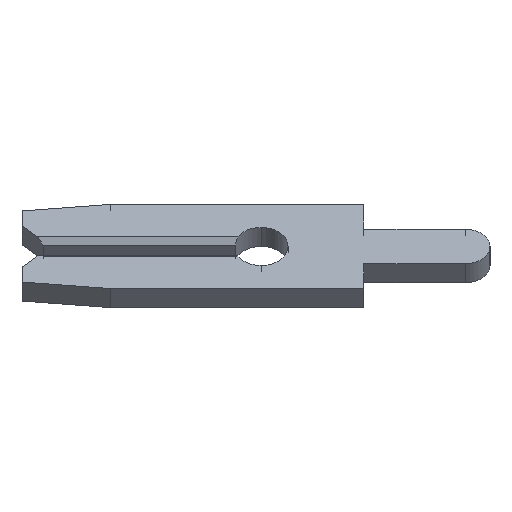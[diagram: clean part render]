
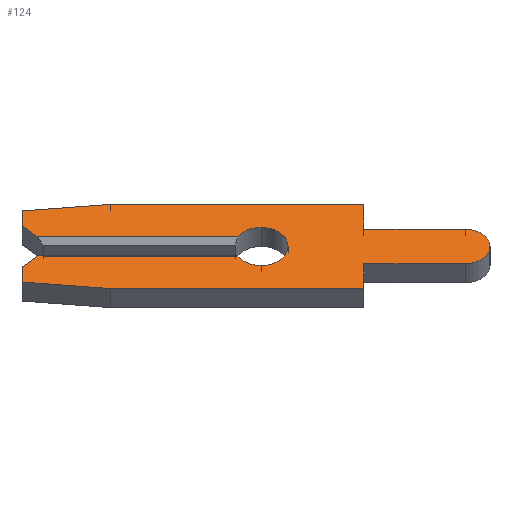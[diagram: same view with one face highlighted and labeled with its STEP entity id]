
A CAD part, left-side view. The second image highlights one B-rep face of the part: STEP entity #124.
In plain terms, the highlighted face is planar.
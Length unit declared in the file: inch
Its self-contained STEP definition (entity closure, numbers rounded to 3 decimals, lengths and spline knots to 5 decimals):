
#3 = DIRECTION ( 'NONE',  ( -1., 0., 0. ) ) ;
#13 = ORIENTED_EDGE ( 'NONE', *, *, #381, .F. ) ;
#19 = VECTOR ( 'NONE', #341, 39.37008 ) ;
#24 = VECTOR ( 'NONE', #311, 39.37008 ) ;
#30 = EDGE_CURVE ( 'NONE', #339, #1290, #826, .T. ) ;
#32 = EDGE_CURVE ( 'NONE', #210, #894, #34, .T. ) ;
#34 = LINE ( 'NONE', #1418, #1035 ) ;
#46 = ORIENTED_EDGE ( 'NONE', *, *, #1098, .F. ) ;
#54 = CARTESIAN_POINT ( 'NONE',  ( -0.013, -0.099, -0.0235 ) ) ;
#84 = VERTEX_POINT ( 'NONE', #255 ) ;
#87 = ORIENTED_EDGE ( 'NONE', *, *, #32, .F. ) ;
#112 = CARTESIAN_POINT ( 'NONE',  ( -0.013, 0.2105, -0.0075 ) ) ;
#122 = VECTOR ( 'NONE', #562, 39.37008 ) ;
#124 = ADVANCED_FACE ( 'NONE', ( #690 ), #1408, .F. ) ;
#150 = ORIENTED_EDGE ( 'NONE', *, *, #1336, .F. ) ;
#151 = ORIENTED_EDGE ( 'NONE', *, *, #1208, .F. ) ;
#154 = EDGE_CURVE ( 'NONE', #354, #579, #536, .T. ) ;
#156 = VECTOR ( 'NONE', #713, 39.37008 ) ;
#170 = EDGE_CURVE ( 'NONE', #1330, #643, #846, .T. ) ;
#190 = VERTEX_POINT ( 'NONE', #397 ) ;
#193 = VERTEX_POINT ( 'NONE', #622 ) ;
#207 = DIRECTION ( 'NONE',  ( 0., -1., 0. ) ) ;
#210 = VERTEX_POINT ( 'NONE', #973 ) ;
#231 = ORIENTED_EDGE ( 'NONE', *, *, #1180, .F. ) ;
#236 = VECTOR ( 'NONE', #1378, 39.37008 ) ;
#253 = CARTESIAN_POINT ( 'NONE',  ( -0.013, 0., 0. ) ) ;
#255 = CARTESIAN_POINT ( 'NONE',  ( -0.013, -0.099, 0.0235 ) ) ;
#258 = CARTESIAN_POINT ( 'NONE',  ( -0.013, 0.231, 0.028 ) ) ;
#273 = LINE ( 'NONE', #1444, #1150 ) ;
#283 = ORIENTED_EDGE ( 'NONE', *, *, #953, .F. ) ;
#287 = CARTESIAN_POINT ( 'NONE',  ( -0.013, 0.231, -0.028 ) ) ;
#300 = ORIENTED_EDGE ( 'NONE', *, *, #1123, .F. ) ;
#311 = DIRECTION ( 'NONE',  ( 0., -1., 0. ) ) ;
#315 = AXIS2_PLACEMENT_3D ( 'NONE', #1159, #366, #591 ) ;
#318 = CARTESIAN_POINT ( 'NONE',  ( -0.013, 0.146, 0.0575 ) ) ;
#321 = VERTEX_POINT ( 'NONE', #769 ) ;
#323 = VERTEX_POINT ( 'NONE', #1216 ) ;
#328 = CARTESIAN_POINT ( 'NONE',  ( -0.013, -0.099, -0.0575 ) ) ;
#331 = LINE ( 'NONE', #991, #24 ) ;
#339 = VERTEX_POINT ( 'NONE', #883 ) ;
#341 = DIRECTION ( 'NONE',  ( 0., 0., -1. ) ) ;
#354 = VERTEX_POINT ( 'NONE', #418 ) ;
#364 = DIRECTION ( 'NONE',  ( -1., 0., 0. ) ) ;
#366 = DIRECTION ( 'NONE',  ( 1., 0., 0. ) ) ;
#368 = CARTESIAN_POINT ( 'NONE',  ( -0.013, 0.02252, 0.013 ) ) ;
#381 = EDGE_CURVE ( 'NONE', #894, #581, #331, .T. ) ;
#385 = DIRECTION ( 'NONE',  ( 0., 1., 0. ) ) ;
#397 = CARTESIAN_POINT ( 'NONE',  ( -0.013, 0.231, -0.028 ) ) ;
#406 = CIRCLE ( 'NONE', #707, 0.026 ) ;
#418 = CARTESIAN_POINT ( 'NONE',  ( -0.013, -0.099, -0.0235 ) ) ;
#441 = EDGE_LOOP ( 'NONE', ( #1400, #151, #283, #300, #1106, #46, #1068, #911, #658, #982, #150, #1461, #875, #938, #13, #87, #231, #1365 ) ) ;
#472 = VECTOR ( 'NONE', #484, 39.37008 ) ;
#474 = DIRECTION ( 'NONE',  ( 0., 0., -1. ) ) ;
#484 = DIRECTION ( 'NONE',  ( 0., 0., 1. ) ) ;
#505 = CARTESIAN_POINT ( 'NONE',  ( -0.013, -0.099, -0.0575 ) ) ;
#515 = AXIS2_PLACEMENT_3D ( 'NONE', #1257, #3, #805 ) ;
#531 = LINE ( 'NONE', #112, #236 ) ;
#535 = EDGE_CURVE ( 'NONE', #1290, #190, #1439, .T. ) ;
#536 = LINE ( 'NONE', #505, #1131 ) ;
#562 = DIRECTION ( 'NONE',  ( 0., -1., 0. ) ) ;
#579 = VERTEX_POINT ( 'NONE', #328 ) ;
#581 = VERTEX_POINT ( 'NONE', #1390 ) ;
#583 = CARTESIAN_POINT ( 'NONE',  ( -0.013, 0.231, -0.04857 ) ) ;
#587 = CARTESIAN_POINT ( 'NONE',  ( -0.013, 0.231, -0.04857 ) ) ;
#591 = DIRECTION ( 'NONE',  ( 0., 0., -1. ) ) ;
#594 = DIRECTION ( 'NONE',  ( 0., 0., 1. ) ) ;
#599 = DIRECTION ( 'NONE',  ( 0., -0.995, 0.105 ) ) ;
#605 = LINE ( 'NONE', #1063, #1291 ) ;
#622 = CARTESIAN_POINT ( 'NONE',  ( -0.013, -0.1975, -0.0235 ) ) ;
#630 = VECTOR ( 'NONE', #1086, 39.37008 ) ;
#635 = EDGE_CURVE ( 'NONE', #1081, #193, #1201, .T. ) ;
#643 = VERTEX_POINT ( 'NONE', #1006 ) ;
#658 = ORIENTED_EDGE ( 'NONE', *, *, #1364, .F. ) ;
#659 = VECTOR ( 'NONE', #207, 39.37008 ) ;
#682 = CARTESIAN_POINT ( 'NONE',  ( -0.013, -0.1975, 0. ) ) ;
#683 = CIRCLE ( 'NONE', #515, 0.026 ) ;
#690 = FACE_OUTER_BOUND ( 'NONE', #441, .T. ) ;
#692 = AXIS2_PLACEMENT_3D ( 'NONE', #711, #1147, #1391 ) ;
#707 = AXIS2_PLACEMENT_3D ( 'NONE', #253, #364, #474 ) ;
#711 = CARTESIAN_POINT ( 'NONE',  ( -0.013, 0., 0. ) ) ;
#713 = DIRECTION ( 'NONE',  ( 0., 0.995, 0.105 ) ) ;
#723 = EDGE_CURVE ( 'NONE', #84, #1081, #1483, .T. ) ;
#733 = DIRECTION ( 'NONE',  ( 0., -1., 0. ) ) ;
#757 = DIRECTION ( 'NONE',  ( 0., 0., 1. ) ) ;
#759 = LINE ( 'NONE', #258, #472 ) ;
#769 = CARTESIAN_POINT ( 'NONE',  ( -0.013, 0.216, -0.013 ) ) ;
#781 = CARTESIAN_POINT ( 'NONE',  ( -0.013, -0.099, 0.0235 ) ) ;
#805 = DIRECTION ( 'NONE',  ( 0., 0., -1. ) ) ;
#813 = CARTESIAN_POINT ( 'NONE',  ( -0.013, -0.099, 0.0575 ) ) ;
#826 = LINE ( 'NONE', #583, #156 ) ;
#846 = LINE ( 'NONE', #857, #1474 ) ;
#857 = CARTESIAN_POINT ( 'NONE',  ( -0.013, 0.2105, 0.0075 ) ) ;
#875 = ORIENTED_EDGE ( 'NONE', *, *, #723, .F. ) ;
#883 = CARTESIAN_POINT ( 'NONE',  ( -0.013, 0.146, -0.0575 ) ) ;
#894 = VERTEX_POINT ( 'NONE', #318 ) ;
#911 = ORIENTED_EDGE ( 'NONE', *, *, #30, .F. ) ;
#938 = ORIENTED_EDGE ( 'NONE', *, *, #1105, .F. ) ;
#945 = LINE ( 'NONE', #54, #630 ) ;
#946 = AXIS2_PLACEMENT_3D ( 'NONE', #682, #1357, #594 ) ;
#953 = EDGE_CURVE ( 'NONE', #323, #972, #956, .T. ) ;
#956 = CIRCLE ( 'NONE', #692, 0.026 ) ;
#972 = VERTEX_POINT ( 'NONE', #1381 ) ;
#973 = CARTESIAN_POINT ( 'NONE',  ( -0.013, 0.231, 0.04857 ) ) ;
#982 = ORIENTED_EDGE ( 'NONE', *, *, #154, .F. ) ;
#991 = CARTESIAN_POINT ( 'NONE',  ( -0.013, 0.146, 0.0575 ) ) ;
#1005 = LINE ( 'NONE', #813, #19 ) ;
#1006 = CARTESIAN_POINT ( 'NONE',  ( -0.013, 0.231, 0.028 ) ) ;
#1017 = VECTOR ( 'NONE', #757, 39.37008 ) ;
#1023 = CARTESIAN_POINT ( 'NONE',  ( -0.013, -0.1975, 0.0235 ) ) ;
#1035 = VECTOR ( 'NONE', #599, 39.37008 ) ;
#1051 = CARTESIAN_POINT ( 'NONE',  ( -0.013, 0.02252, -0.013 ) ) ;
#1063 = CARTESIAN_POINT ( 'NONE',  ( -0.013, 0., -0.013 ) ) ;
#1068 = ORIENTED_EDGE ( 'NONE', *, *, #535, .F. ) ;
#1081 = VERTEX_POINT ( 'NONE', #1023 ) ;
#1086 = DIRECTION ( 'NONE',  ( 0., 1., 0. ) ) ;
#1090 = EDGE_CURVE ( 'NONE', #1330, #1286, #1425, .T. ) ;
#1098 = EDGE_CURVE ( 'NONE', #190, #321, #531, .T. ) ;
#1105 = EDGE_CURVE ( 'NONE', #581, #84, #1005, .T. ) ;
#1106 = ORIENTED_EDGE ( 'NONE', *, *, #1176, .F. ) ;
#1123 = EDGE_CURVE ( 'NONE', #1249, #323, #683, .T. ) ;
#1131 = VECTOR ( 'NONE', #1426, 39.37008 ) ;
#1147 = DIRECTION ( 'NONE',  ( -1., 0., 0. ) ) ;
#1150 = VECTOR ( 'NONE', #385, 39.37008 ) ;
#1159 = CARTESIAN_POINT ( 'NONE',  ( -0.013, 0., 0. ) ) ;
#1161 = CARTESIAN_POINT ( 'NONE',  ( -0.013, 0.231, 0.013 ) ) ;
#1176 = EDGE_CURVE ( 'NONE', #321, #1249, #605, .T. ) ;
#1180 = EDGE_CURVE ( 'NONE', #643, #210, #759, .T. ) ;
#1201 = CIRCLE ( 'NONE', #946, 0.0235 ) ;
#1208 = EDGE_CURVE ( 'NONE', #972, #1286, #406, .T. ) ;
#1212 = CARTESIAN_POINT ( 'NONE',  ( -0.013, 0.216, 0.013 ) ) ;
#1216 = CARTESIAN_POINT ( 'NONE',  ( -0.013, 0., -0.026 ) ) ;
#1249 = VERTEX_POINT ( 'NONE', #1051 ) ;
#1257 = CARTESIAN_POINT ( 'NONE',  ( -0.013, 0., 0. ) ) ;
#1286 = VERTEX_POINT ( 'NONE', #368 ) ;
#1290 = VERTEX_POINT ( 'NONE', #587 ) ;
#1291 = VECTOR ( 'NONE', #733, 39.37008 ) ;
#1324 = DIRECTION ( 'NONE',  ( 0., 0.707, 0.707 ) ) ;
#1330 = VERTEX_POINT ( 'NONE', #1212 ) ;
#1336 = EDGE_CURVE ( 'NONE', #193, #354, #945, .T. ) ;
#1357 = DIRECTION ( 'NONE',  ( 1., 0., 0. ) ) ;
#1364 = EDGE_CURVE ( 'NONE', #579, #339, #273, .T. ) ;
#1365 = ORIENTED_EDGE ( 'NONE', *, *, #170, .F. ) ;
#1378 = DIRECTION ( 'NONE',  ( 0., -0.707, 0.707 ) ) ;
#1381 = CARTESIAN_POINT ( 'NONE',  ( -0.013, 0., 0.026 ) ) ;
#1390 = CARTESIAN_POINT ( 'NONE',  ( -0.013, -0.099, 0.0575 ) ) ;
#1391 = DIRECTION ( 'NONE',  ( 0., 0., -1. ) ) ;
#1400 = ORIENTED_EDGE ( 'NONE', *, *, #1090, .T. ) ;
#1408 = PLANE ( 'NONE',  #315 ) ;
#1418 = CARTESIAN_POINT ( 'NONE',  ( -0.013, 0.231, 0.04857 ) ) ;
#1425 = LINE ( 'NONE', #1161, #122 ) ;
#1426 = DIRECTION ( 'NONE',  ( 0., 0., -1. ) ) ;
#1439 = LINE ( 'NONE', #287, #1017 ) ;
#1444 = CARTESIAN_POINT ( 'NONE',  ( -0.013, 0.146, -0.0575 ) ) ;
#1461 = ORIENTED_EDGE ( 'NONE', *, *, #635, .F. ) ;
#1474 = VECTOR ( 'NONE', #1324, 39.37008 ) ;
#1483 = LINE ( 'NONE', #781, #659 ) ;
